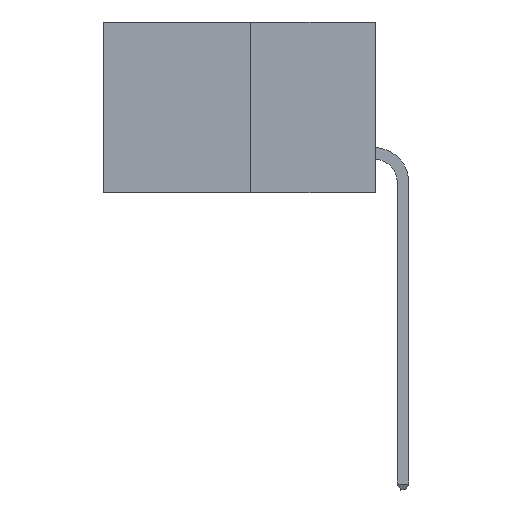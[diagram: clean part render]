
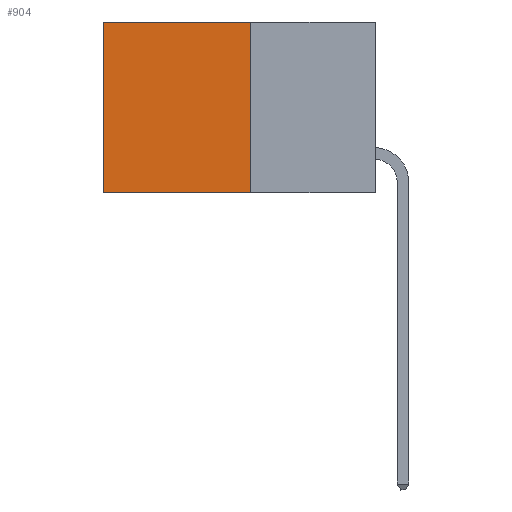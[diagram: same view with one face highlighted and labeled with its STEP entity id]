
A CAD part, left-side view. The second image highlights one B-rep face of the part: STEP entity #904.
In plain terms, the highlighted planar face has unit normal (-1, 0, 0).
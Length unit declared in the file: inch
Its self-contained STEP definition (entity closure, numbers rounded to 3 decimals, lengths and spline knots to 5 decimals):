
#904 = ADVANCED_FACE ( 'NONE', ( #2313 ), #12530, .F. ) ;
#1616 = VERTEX_POINT ( 'NONE', #2484 ) ;
#1690 = ORIENTED_EDGE ( 'NONE', *, *, #2469, .T. ) ;
#2058 = ORIENTED_EDGE ( 'NONE', *, *, #2663, .T. ) ;
#2313 = FACE_OUTER_BOUND ( 'NONE', #13497, .T. ) ;
#2469 = EDGE_CURVE ( 'NONE', #4511, #3604, #2998, .T. ) ;
#2484 = CARTESIAN_POINT ( 'NONE',  ( 0.277, 0.27, -0.37 ) ) ;
#2663 = EDGE_CURVE ( 'NONE', #13247, #4511, #6694, .T. ) ;
#2979 = LINE ( 'NONE', #9596, #8429 ) ;
#2998 = LINE ( 'NONE', #5590, #8823 ) ;
#3304 = CARTESIAN_POINT ( 'NONE',  ( 0.277, 0.27, 0. ) ) ;
#3427 = EDGE_CURVE ( 'NONE', #1616, #3604, #4092, .T. ) ;
#3604 = VERTEX_POINT ( 'NONE', #10172 ) ;
#3717 = DIRECTION ( 'NONE',  ( 1., 0., 0. ) ) ;
#4092 = LINE ( 'NONE', #10605, #6834 ) ;
#4511 = VERTEX_POINT ( 'NONE', #9604 ) ;
#4823 = CARTESIAN_POINT ( 'NONE',  ( 0.277, 0.27, -0.37 ) ) ;
#4833 = ORIENTED_EDGE ( 'NONE', *, *, #3427, .F. ) ;
#5590 = CARTESIAN_POINT ( 'NONE',  ( 0.277, 0.59, -0.37 ) ) ;
#5965 = VECTOR ( 'NONE', #12159, 39.37008 ) ;
#6694 = LINE ( 'NONE', #12146, #5965 ) ;
#6834 = VECTOR ( 'NONE', #12346, 39.37008 ) ;
#8429 = VECTOR ( 'NONE', #8461, 39.37008 ) ;
#8461 = DIRECTION ( 'NONE',  ( 0., 0., -1. ) ) ;
#8823 = VECTOR ( 'NONE', #10206, 39.37008 ) ;
#9596 = CARTESIAN_POINT ( 'NONE',  ( 0.277, 0.27, -0.37 ) ) ;
#9604 = CARTESIAN_POINT ( 'NONE',  ( 0.277, 0.59, 0. ) ) ;
#10069 = AXIS2_PLACEMENT_3D ( 'NONE', #4823, #3717, #12822 ) ;
#10172 = CARTESIAN_POINT ( 'NONE',  ( 0.277, 0.59, -0.37 ) ) ;
#10206 = DIRECTION ( 'NONE',  ( 0., 0., -1. ) ) ;
#10605 = CARTESIAN_POINT ( 'NONE',  ( 0.277, 0.27, -0.37 ) ) ;
#10844 = ORIENTED_EDGE ( 'NONE', *, *, #12137, .F. ) ;
#12137 = EDGE_CURVE ( 'NONE', #13247, #1616, #2979, .T. ) ;
#12146 = CARTESIAN_POINT ( 'NONE',  ( 0.277, 0.27, 0. ) ) ;
#12159 = DIRECTION ( 'NONE',  ( 0., 1., 0. ) ) ;
#12346 = DIRECTION ( 'NONE',  ( 0., 1., 0. ) ) ;
#12530 = PLANE ( 'NONE',  #10069 ) ;
#12822 = DIRECTION ( 'NONE',  ( 0., 0., -1. ) ) ;
#13247 = VERTEX_POINT ( 'NONE', #3304 ) ;
#13497 = EDGE_LOOP ( 'NONE', ( #1690, #4833, #10844, #2058 ) ) ;
